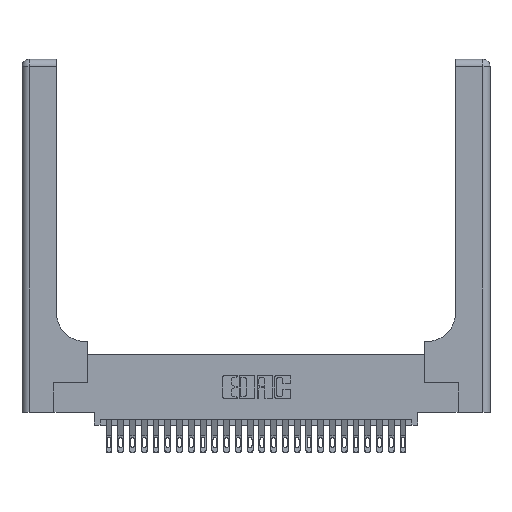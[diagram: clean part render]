
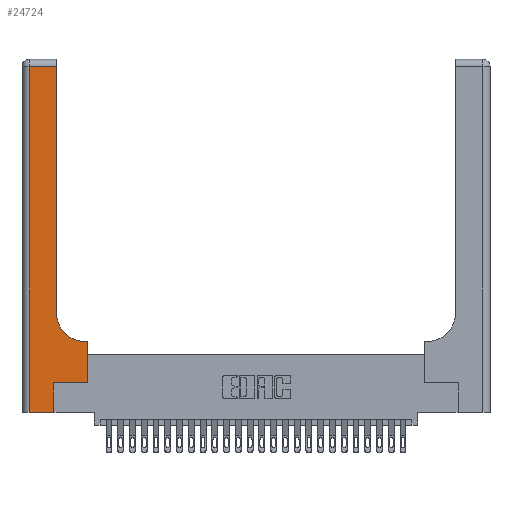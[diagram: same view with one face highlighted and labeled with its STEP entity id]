
A CAD part, top view. The second image highlights one B-rep face of the part: STEP entity #24724.
In plain terms, the highlighted planar face has unit normal (0, 0, 1).
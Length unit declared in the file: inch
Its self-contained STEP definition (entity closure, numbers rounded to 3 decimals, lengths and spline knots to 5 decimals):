
#209 = ORIENTED_EDGE ( 'NONE', *, *, #3325, .T. ) ;
#425 = ORIENTED_EDGE ( 'NONE', *, *, #26272, .T. ) ;
#454 = EDGE_CURVE ( 'NONE', #24487, #14655, #27771, .T. ) ;
#723 = LINE ( 'NONE', #14271, #11602 ) ;
#1595 = DIRECTION ( 'NONE',  ( 1., 0., 0. ) ) ;
#1887 = VECTOR ( 'NONE', #1595, 39.37008 ) ;
#2076 = DIRECTION ( 'NONE',  ( 0., 0., -1. ) ) ;
#2490 = CARTESIAN_POINT ( 'NONE',  ( 0.269, 0., 0.37 ) ) ;
#2636 = EDGE_CURVE ( 'NONE', #3405, #17592, #11601, .T. ) ;
#2699 = CARTESIAN_POINT ( 'NONE',  ( 0.2915, 2.94, 0.37 ) ) ;
#2851 = VECTOR ( 'NONE', #8477, 39.37008 ) ;
#3325 = EDGE_CURVE ( 'NONE', #20953, #4537, #15475, .T. ) ;
#3405 = VERTEX_POINT ( 'NONE', #7276 ) ;
#3465 = DIRECTION ( 'NONE',  ( 1., 0., 0. ) ) ;
#4146 = VECTOR ( 'NONE', #20805, 39.37008 ) ;
#4432 = AXIS2_PLACEMENT_3D ( 'NONE', #28133, #2076, #17259 ) ;
#4537 = VERTEX_POINT ( 'NONE', #2699 ) ;
#4779 = LINE ( 'NONE', #6594, #8862 ) ;
#5819 = VECTOR ( 'NONE', #23694, 39.37008 ) ;
#6164 = CARTESIAN_POINT ( 'NONE',  ( 0.269, 0.25, 0.37 ) ) ;
#6172 = LINE ( 'NONE', #14582, #4146 ) ;
#6594 = CARTESIAN_POINT ( 'NONE',  ( 0.2915, 0.6, 0.37 ) ) ;
#6864 = ORIENTED_EDGE ( 'NONE', *, *, #16473, .T. ) ;
#7276 = CARTESIAN_POINT ( 'NONE',  ( 0.269, 0.25, 0.37 ) ) ;
#8477 = DIRECTION ( 'NONE',  ( 0., -1., 0. ) ) ;
#8691 = VECTOR ( 'NONE', #24863, 39.37008 ) ;
#8862 = VECTOR ( 'NONE', #19812, 39.37008 ) ;
#9002 = CARTESIAN_POINT ( 'NONE',  ( 0.5415, 0.6, 0.37 ) ) ;
#9039 = VERTEX_POINT ( 'NONE', #9002 ) ;
#9418 = CIRCLE ( 'NONE', #23737, 0.25 ) ;
#10010 = DIRECTION ( 'NONE',  ( 0., 1., 0. ) ) ;
#10987 = CARTESIAN_POINT ( 'NONE',  ( 0.5585, 0.25, 0.37 ) ) ;
#11580 = ORIENTED_EDGE ( 'NONE', *, *, #2636, .T. ) ;
#11601 = LINE ( 'NONE', #6164, #5819 ) ;
#11602 = VECTOR ( 'NONE', #10010, 39.37008 ) ;
#12735 = ORIENTED_EDGE ( 'NONE', *, *, #28190, .T. ) ;
#12884 = PLANE ( 'NONE',  #4432 ) ;
#13588 = CARTESIAN_POINT ( 'NONE',  ( 0.2915, 0.85, 0.37 ) ) ;
#14271 = CARTESIAN_POINT ( 'NONE',  ( 0.5585, 0.25, 0.37 ) ) ;
#14582 = CARTESIAN_POINT ( 'NONE',  ( 0.269, 0., 0.37 ) ) ;
#14655 = VERTEX_POINT ( 'NONE', #2490 ) ;
#15023 = ORIENTED_EDGE ( 'NONE', *, *, #454, .T. ) ;
#15393 = ORIENTED_EDGE ( 'NONE', *, *, #21834, .T. ) ;
#15475 = LINE ( 'NONE', #26964, #8691 ) ;
#16087 = FACE_OUTER_BOUND ( 'NONE', #27600, .T. ) ;
#16369 = ORIENTED_EDGE ( 'NONE', *, *, #19957, .T. ) ;
#16473 = EDGE_CURVE ( 'NONE', #17601, #24487, #21588, .T. ) ;
#17259 = DIRECTION ( 'NONE',  ( -1., 0., 0. ) ) ;
#17592 = VERTEX_POINT ( 'NONE', #10987 ) ;
#17601 = VERTEX_POINT ( 'NONE', #19744 ) ;
#17611 = VECTOR ( 'NONE', #20661, 39.37008 ) ;
#18312 = LINE ( 'NONE', #22686, #17611 ) ;
#18996 = CARTESIAN_POINT ( 'NONE',  ( 0., 0., 0.37 ) ) ;
#19744 = CARTESIAN_POINT ( 'NONE',  ( 0.06, 2.94, 0.37 ) ) ;
#19812 = DIRECTION ( 'NONE',  ( -1., 0., 0. ) ) ;
#19957 = EDGE_CURVE ( 'NONE', #23907, #9039, #4779, .T. ) ;
#20661 = DIRECTION ( 'NONE',  ( -1., 0., 0. ) ) ;
#20805 = DIRECTION ( 'NONE',  ( 0., 1., 0. ) ) ;
#20953 = VERTEX_POINT ( 'NONE', #13588 ) ;
#21546 = CARTESIAN_POINT ( 'NONE',  ( 0.06, 3., 0.37 ) ) ;
#21588 = LINE ( 'NONE', #21546, #2851 ) ;
#21834 = EDGE_CURVE ( 'NONE', #9039, #20953, #9418, .T. ) ;
#22686 = CARTESIAN_POINT ( 'NONE',  ( 0., 2.94, 0.37 ) ) ;
#22831 = ORIENTED_EDGE ( 'NONE', *, *, #25752, .T. ) ;
#22887 = DIRECTION ( 'NONE',  ( 0., 0., -1. ) ) ;
#23694 = DIRECTION ( 'NONE',  ( 1., 0., 0. ) ) ;
#23737 = AXIS2_PLACEMENT_3D ( 'NONE', #27259, #22887, #3465 ) ;
#23907 = VERTEX_POINT ( 'NONE', #23979 ) ;
#23979 = CARTESIAN_POINT ( 'NONE',  ( 0.5585, 0.6, 0.37 ) ) ;
#24487 = VERTEX_POINT ( 'NONE', #25670 ) ;
#24724 = ADVANCED_FACE ( 'NONE', ( #16087 ), #12884, .F. ) ;
#24863 = DIRECTION ( 'NONE',  ( 0., 1., 0. ) ) ;
#25670 = CARTESIAN_POINT ( 'NONE',  ( 0.06, 0., 0.37 ) ) ;
#25752 = EDGE_CURVE ( 'NONE', #14655, #3405, #6172, .T. ) ;
#26272 = EDGE_CURVE ( 'NONE', #17592, #23907, #723, .T. ) ;
#26964 = CARTESIAN_POINT ( 'NONE',  ( 0.2915, 3., 0.37 ) ) ;
#27259 = CARTESIAN_POINT ( 'NONE',  ( 0.5415, 0.85, 0.37 ) ) ;
#27600 = EDGE_LOOP ( 'NONE', ( #209, #12735, #6864, #15023, #22831, #11580, #425, #16369, #15393 ) ) ;
#27771 = LINE ( 'NONE', #18996, #1887 ) ;
#28133 = CARTESIAN_POINT ( 'NONE',  ( 0., 3., 0.37 ) ) ;
#28190 = EDGE_CURVE ( 'NONE', #4537, #17601, #18312, .T. ) ;
